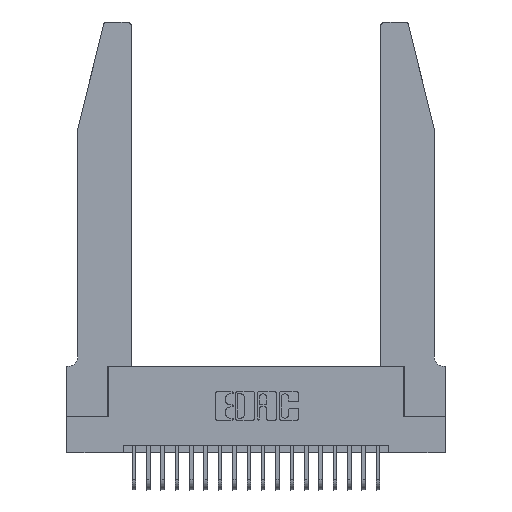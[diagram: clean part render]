
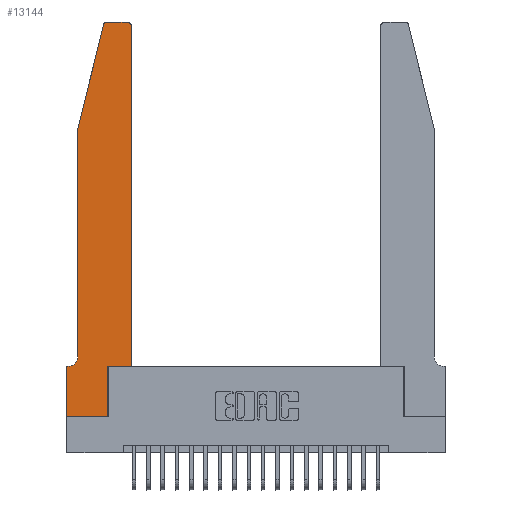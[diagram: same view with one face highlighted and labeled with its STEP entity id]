
A CAD part, top view. The second image highlights one B-rep face of the part: STEP entity #13144.
In plain terms, the highlighted planar face has unit normal (0, 0, 1).
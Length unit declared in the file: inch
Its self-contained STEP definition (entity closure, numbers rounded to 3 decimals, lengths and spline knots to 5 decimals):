
#26 = PLANE ( 'NONE',  #23226 ) ;
#622 = CARTESIAN_POINT ( 'NONE',  ( 0.2865, 0., 0.37 ) ) ;
#630 = ORIENTED_EDGE ( 'NONE', *, *, #23224, .T. ) ;
#684 = ORIENTED_EDGE ( 'NONE', *, *, #1839, .T. ) ;
#1142 = LINE ( 'NONE', #8315, #10075 ) ;
#1341 = AXIS2_PLACEMENT_3D ( 'NONE', #16423, #13023, #22271 ) ;
#1435 = VERTEX_POINT ( 'NONE', #14150 ) ;
#1437 = CARTESIAN_POINT ( 'NONE',  ( 0., 0., 0.37 ) ) ;
#1475 = LINE ( 'NONE', #1437, #6090 ) ;
#1839 = EDGE_CURVE ( 'NONE', #22350, #14143, #4171, .T. ) ;
#2315 = DIRECTION ( 'NONE',  ( 1., 0., 0. ) ) ;
#2411 = VECTOR ( 'NONE', #20874, 39.37008 ) ;
#2618 = EDGE_CURVE ( 'NONE', #6197, #22883, #22260, .T. ) ;
#2719 = DIRECTION ( 'NONE',  ( -1., 0., 0. ) ) ;
#3374 = ORIENTED_EDGE ( 'NONE', *, *, #18447, .T. ) ;
#3880 = DIRECTION ( 'NONE',  ( -0.239, -0.971, 0. ) ) ;
#4171 = CIRCLE ( 'NONE', #16457, 0.03 ) ;
#4504 = CARTESIAN_POINT ( 'NONE',  ( 0.0755, 2., 0.37 ) ) ;
#4735 = VECTOR ( 'NONE', #2719, 39.37008 ) ;
#4859 = DIRECTION ( 'NONE',  ( -1., 0., 0. ) ) ;
#5036 = LINE ( 'NONE', #17093, #4735 ) ;
#6090 = VECTOR ( 'NONE', #2315, 39.37008 ) ;
#6121 = LINE ( 'NONE', #21567, #19336 ) ;
#6189 = CARTESIAN_POINT ( 'NONE',  ( 0.2865, 0.35, 0.37 ) ) ;
#6197 = VERTEX_POINT ( 'NONE', #17401 ) ;
#6726 = ORIENTED_EDGE ( 'NONE', *, *, #2618, .T. ) ;
#6881 = LINE ( 'NONE', #9814, #7186 ) ;
#7066 = EDGE_LOOP ( 'NONE', ( #3374, #19859, #18671, #16131, #630, #14271, #10972, #13227, #19513, #6726, #10251, #684 ) ) ;
#7186 = VECTOR ( 'NONE', #13172, 39.37008 ) ;
#8315 = CARTESIAN_POINT ( 'NONE',  ( 0.4505, 0.35, 0.37 ) ) ;
#8410 = DIRECTION ( 'NONE',  ( 1., 0., 0. ) ) ;
#8575 = CARTESIAN_POINT ( 'NONE',  ( 0.4505, 0.35, 0.37 ) ) ;
#8960 = CARTESIAN_POINT ( 'NONE',  ( 0.0055, 0.35, 0.37 ) ) ;
#9814 = CARTESIAN_POINT ( 'NONE',  ( 0.0755, 2., 0.37 ) ) ;
#9972 = FACE_OUTER_BOUND ( 'NONE', #7066, .T. ) ;
#10075 = VECTOR ( 'NONE', #19272, 39.37008 ) ;
#10215 = CARTESIAN_POINT ( 'NONE',  ( 0.4205, 2.75, 0.37 ) ) ;
#10251 = ORIENTED_EDGE ( 'NONE', *, *, #20065, .T. ) ;
#10373 = EDGE_CURVE ( 'NONE', #1435, #12094, #1475, .T. ) ;
#10801 = CARTESIAN_POINT ( 'NONE',  ( 0.284, 2.72, 0.37 ) ) ;
#10909 = CARTESIAN_POINT ( 'NONE',  ( 0.4505, 0.35, 0.37 ) ) ;
#10972 = ORIENTED_EDGE ( 'NONE', *, *, #16247, .T. ) ;
#10982 = DIRECTION ( 'NONE',  ( 0., 0., 1. ) ) ;
#11588 = CARTESIAN_POINT ( 'NONE',  ( 0., 0.35, 0.37 ) ) ;
#12094 = VERTEX_POINT ( 'NONE', #622 ) ;
#12121 = EDGE_CURVE ( 'NONE', #13483, #14492, #6881, .T. ) ;
#12134 = CARTESIAN_POINT ( 'NONE',  ( 0.25487, 2.72718, 0.37 ) ) ;
#12634 = DIRECTION ( 'NONE',  ( 1., 0., 0. ) ) ;
#12848 = CARTESIAN_POINT ( 'NONE',  ( 0.0755, 0.42, 0.37 ) ) ;
#13023 = DIRECTION ( 'NONE',  ( 0., 0., -1. ) ) ;
#13144 = ADVANCED_FACE ( 'NONE', ( #9972 ), #26, .T. ) ;
#13172 = DIRECTION ( 'NONE',  ( 0., -1., 0. ) ) ;
#13227 = ORIENTED_EDGE ( 'NONE', *, *, #10373, .T. ) ;
#13483 = VERTEX_POINT ( 'NONE', #4504 ) ;
#13517 = VERTEX_POINT ( 'NONE', #11588 ) ;
#13758 = AXIS2_PLACEMENT_3D ( 'NONE', #10801, #18159, #19911 ) ;
#13851 = DIRECTION ( 'NONE',  ( 1., 0., 0. ) ) ;
#13928 = VECTOR ( 'NONE', #8410, 39.37008 ) ;
#14143 = VERTEX_POINT ( 'NONE', #10215 ) ;
#14150 = CARTESIAN_POINT ( 'NONE',  ( 0., 0., 0.37 ) ) ;
#14271 = ORIENTED_EDGE ( 'NONE', *, *, #22617, .T. ) ;
#14304 = CARTESIAN_POINT ( 'NONE',  ( 0.4505, 2.72, 0.37 ) ) ;
#14486 = CIRCLE ( 'NONE', #1341, 0.07 ) ;
#14492 = VERTEX_POINT ( 'NONE', #12848 ) ;
#14809 = CARTESIAN_POINT ( 'NONE',  ( 0.0755, 2., 0.37 ) ) ;
#14949 = DIRECTION ( 'NONE',  ( 0., -1., 0. ) ) ;
#15427 = CARTESIAN_POINT ( 'NONE',  ( 0.284, 2.75, 0.37 ) ) ;
#15700 = CARTESIAN_POINT ( 'NONE',  ( 0.4205, 2.72, 0.37 ) ) ;
#15956 = VECTOR ( 'NONE', #14949, 39.37008 ) ;
#16131 = ORIENTED_EDGE ( 'NONE', *, *, #12121, .T. ) ;
#16173 = LINE ( 'NONE', #14809, #18744 ) ;
#16247 = EDGE_CURVE ( 'NONE', #13517, #1435, #16543, .T. ) ;
#16423 = CARTESIAN_POINT ( 'NONE',  ( 0.0055, 0.42, 0.37 ) ) ;
#16457 = AXIS2_PLACEMENT_3D ( 'NONE', #15700, #19232, #13851 ) ;
#16543 = LINE ( 'NONE', #22263, #15956 ) ;
#17093 = CARTESIAN_POINT ( 'NONE',  ( 0.0755, 0.35, 0.37 ) ) ;
#17401 = CARTESIAN_POINT ( 'NONE',  ( 0.2865, 0.35, 0.37 ) ) ;
#17915 = LINE ( 'NONE', #6189, #2411 ) ;
#18159 = DIRECTION ( 'NONE',  ( 0., 0., 1. ) ) ;
#18447 = EDGE_CURVE ( 'NONE', #14143, #20284, #6121, .T. ) ;
#18671 = ORIENTED_EDGE ( 'NONE', *, *, #18689, .T. ) ;
#18689 = EDGE_CURVE ( 'NONE', #23720, #13483, #16173, .T. ) ;
#18744 = VECTOR ( 'NONE', #3880, 39.37008 ) ;
#19095 = EDGE_CURVE ( 'NONE', #20284, #23720, #19290, .T. ) ;
#19198 = VERTEX_POINT ( 'NONE', #8960 ) ;
#19232 = DIRECTION ( 'NONE',  ( 0., 0., 1. ) ) ;
#19272 = DIRECTION ( 'NONE',  ( 0., 1., 0. ) ) ;
#19290 = CIRCLE ( 'NONE', #13758, 0.03 ) ;
#19336 = VECTOR ( 'NONE', #4859, 39.37008 ) ;
#19513 = ORIENTED_EDGE ( 'NONE', *, *, #23516, .T. ) ;
#19859 = ORIENTED_EDGE ( 'NONE', *, *, #19095, .T. ) ;
#19911 = DIRECTION ( 'NONE',  ( 1., 0., 0. ) ) ;
#20065 = EDGE_CURVE ( 'NONE', #22883, #22350, #1142, .T. ) ;
#20284 = VERTEX_POINT ( 'NONE', #15427 ) ;
#20874 = DIRECTION ( 'NONE',  ( 0., 1., 0. ) ) ;
#21567 = CARTESIAN_POINT ( 'NONE',  ( 0.2605, 2.75, 0.37 ) ) ;
#21957 = CARTESIAN_POINT ( 'NONE',  ( 0., 0.35, 0.37 ) ) ;
#22260 = LINE ( 'NONE', #8575, #13928 ) ;
#22263 = CARTESIAN_POINT ( 'NONE',  ( 0., 0., 0.37 ) ) ;
#22271 = DIRECTION ( 'NONE',  ( -1., 0., 0. ) ) ;
#22350 = VERTEX_POINT ( 'NONE', #14304 ) ;
#22617 = EDGE_CURVE ( 'NONE', #19198, #13517, #5036, .T. ) ;
#22883 = VERTEX_POINT ( 'NONE', #10909 ) ;
#23224 = EDGE_CURVE ( 'NONE', #14492, #19198, #14486, .T. ) ;
#23226 = AXIS2_PLACEMENT_3D ( 'NONE', #21957, #10982, #12634 ) ;
#23516 = EDGE_CURVE ( 'NONE', #12094, #6197, #17915, .T. ) ;
#23720 = VERTEX_POINT ( 'NONE', #12134 ) ;
